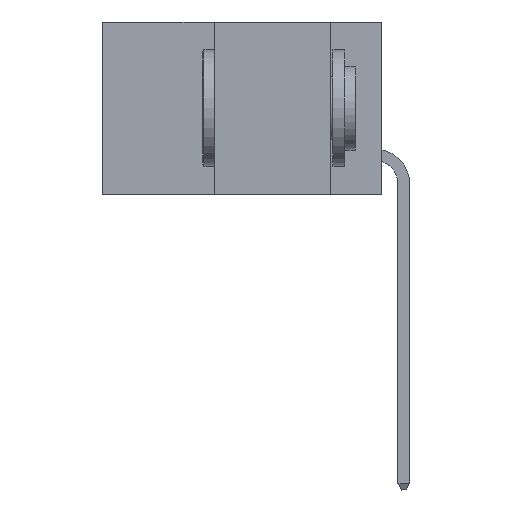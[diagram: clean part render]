
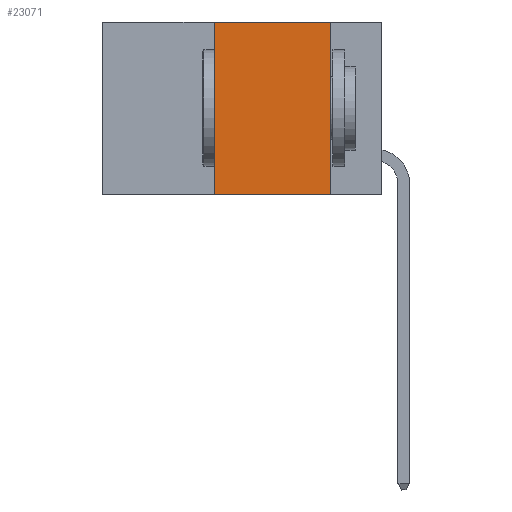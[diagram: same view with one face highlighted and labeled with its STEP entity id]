
A CAD part, left-side view. The second image highlights one B-rep face of the part: STEP entity #23071.
In plain terms, the highlighted planar face has unit normal (-1, 0, 0).
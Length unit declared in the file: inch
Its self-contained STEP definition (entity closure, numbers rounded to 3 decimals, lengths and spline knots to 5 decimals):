
#1115 = CARTESIAN_POINT ( 'NONE',  ( 0., 0.11, 0. ) ) ;
#3152 = DIRECTION ( 'NONE',  ( 0., 0., -1. ) ) ;
#4950 = CARTESIAN_POINT ( 'NONE',  ( 0., 0.6, 0. ) ) ;
#8569 = VERTEX_POINT ( 'NONE', #36416 ) ;
#11281 = DIRECTION ( 'NONE',  ( 0., 0., 1. ) ) ;
#11413 = DIRECTION ( 'NONE',  ( 0., 0., -1. ) ) ;
#14071 = FACE_OUTER_BOUND ( 'NONE', #34430, .T. ) ;
#14382 = CARTESIAN_POINT ( 'NONE',  ( 0., 0.6, 0. ) ) ;
#14701 = LINE ( 'NONE', #44179, #39676 ) ;
#14754 = VECTOR ( 'NONE', #35768, 39.37008 ) ;
#15461 = VERTEX_POINT ( 'NONE', #30283 ) ;
#18378 = DIRECTION ( 'NONE',  ( 1., 0., 0. ) ) ;
#19521 = EDGE_CURVE ( 'NONE', #8569, #15461, #33398, .T. ) ;
#21117 = VECTOR ( 'NONE', #11281, 39.37008 ) ;
#23071 = ADVANCED_FACE ( 'NONE', ( #14071 ), #25183, .F. ) ;
#23719 = ORIENTED_EDGE ( 'NONE', *, *, #19521, .T. ) ;
#25053 = CARTESIAN_POINT ( 'NONE',  ( 0., 0.36, 0. ) ) ;
#25183 = PLANE ( 'NONE',  #34141 ) ;
#26542 = LINE ( 'NONE', #25053, #21117 ) ;
#28345 = VERTEX_POINT ( 'NONE', #1115 ) ;
#28427 = CARTESIAN_POINT ( 'NONE',  ( 0., 0.6, -0.37 ) ) ;
#30283 = CARTESIAN_POINT ( 'NONE',  ( 0., 0.11, -0.37 ) ) ;
#31158 = EDGE_CURVE ( 'NONE', #28345, #15461, #14701, .T. ) ;
#33398 = LINE ( 'NONE', #28427, #39370 ) ;
#34141 = AXIS2_PLACEMENT_3D ( 'NONE', #4950, #18378, #11413 ) ;
#34430 = EDGE_LOOP ( 'NONE', ( #40723, #37256, #35146, #23719 ) ) ;
#35146 = ORIENTED_EDGE ( 'NONE', *, *, #43979, .F. ) ;
#35768 = DIRECTION ( 'NONE',  ( 0., -1., 0. ) ) ;
#36416 = CARTESIAN_POINT ( 'NONE',  ( 0., 0.36, -0.37 ) ) ;
#37256 = ORIENTED_EDGE ( 'NONE', *, *, #42266, .F. ) ;
#38749 = DIRECTION ( 'NONE',  ( 0., -1., 0. ) ) ;
#39370 = VECTOR ( 'NONE', #38749, 39.37008 ) ;
#39676 = VECTOR ( 'NONE', #3152, 39.37008 ) ;
#39738 = LINE ( 'NONE', #14382, #14754 ) ;
#40723 = ORIENTED_EDGE ( 'NONE', *, *, #31158, .F. ) ;
#42206 = VERTEX_POINT ( 'NONE', #42434 ) ;
#42266 = EDGE_CURVE ( 'NONE', #42206, #28345, #39738, .T. ) ;
#42434 = CARTESIAN_POINT ( 'NONE',  ( 0., 0.36, 0. ) ) ;
#43979 = EDGE_CURVE ( 'NONE', #8569, #42206, #26542, .T. ) ;
#44179 = CARTESIAN_POINT ( 'NONE',  ( 0., 0.11, 0. ) ) ;
